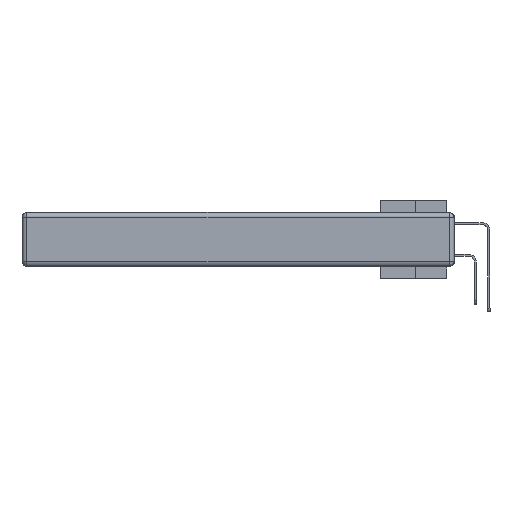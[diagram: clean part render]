
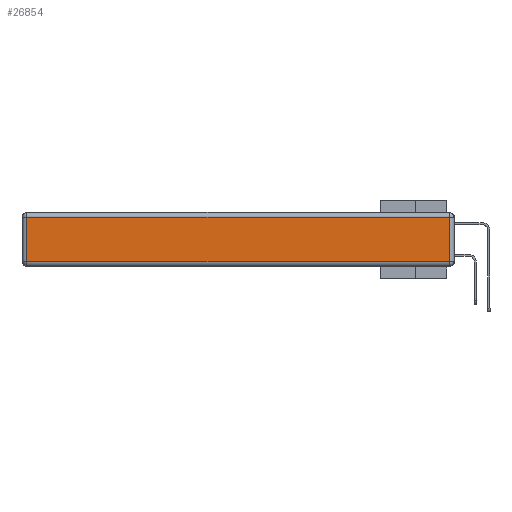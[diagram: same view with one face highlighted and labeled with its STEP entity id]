
A CAD part, left-side view. The second image highlights one B-rep face of the part: STEP entity #26854.
In plain terms, the highlighted planar face has unit normal (-1, 0, 0).
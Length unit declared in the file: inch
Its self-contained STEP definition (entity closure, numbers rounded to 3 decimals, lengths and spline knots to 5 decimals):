
#934 = VECTOR ( 'NONE', #37594, 39.37008 ) ;
#1810 = ORIENTED_EDGE ( 'NONE', *, *, #22919, .T. ) ;
#3829 = CARTESIAN_POINT ( 'NONE',  ( 0., 0.03, -0.03 ) ) ;
#5881 = FACE_OUTER_BOUND ( 'NONE', #35459, .T. ) ;
#6010 = CARTESIAN_POINT ( 'NONE',  ( 0., 2.72, -0.343 ) ) ;
#8460 = CARTESIAN_POINT ( 'NONE',  ( 0., 2.72, -0.03 ) ) ;
#8880 = CARTESIAN_POINT ( 'NONE',  ( 0., 0.03, -0.313 ) ) ;
#9746 = EDGE_CURVE ( 'NONE', #11923, #16937, #11888, .T. ) ;
#10973 = LINE ( 'NONE', #36894, #29405 ) ;
#11493 = DIRECTION ( 'NONE',  ( 0., -1., 0. ) ) ;
#11888 = LINE ( 'NONE', #37583, #28739 ) ;
#11923 = VERTEX_POINT ( 'NONE', #3829 ) ;
#13041 = PLANE ( 'NONE',  #17216 ) ;
#14494 = VECTOR ( 'NONE', #11493, 39.37008 ) ;
#15268 = DIRECTION ( 'NONE',  ( 0., 1., 0. ) ) ;
#16937 = VERTEX_POINT ( 'NONE', #8460 ) ;
#17216 = AXIS2_PLACEMENT_3D ( 'NONE', #31543, #19126, #37862 ) ;
#19126 = DIRECTION ( 'NONE',  ( -1., 0., 0. ) ) ;
#22044 = ORIENTED_EDGE ( 'NONE', *, *, #9746, .T. ) ;
#22919 = EDGE_CURVE ( 'NONE', #16937, #31050, #37797, .T. ) ;
#23920 = LINE ( 'NONE', #30861, #14494 ) ;
#24719 = CARTESIAN_POINT ( 'NONE',  ( 0., 2.72, -0.313 ) ) ;
#25894 = ORIENTED_EDGE ( 'NONE', *, *, #26064, .T. ) ;
#26064 = EDGE_CURVE ( 'NONE', #31050, #36430, #23920, .T. ) ;
#26854 = ADVANCED_FACE ( 'NONE', ( #5881 ), #13041, .T. ) ;
#28739 = VECTOR ( 'NONE', #15268, 39.37008 ) ;
#29405 = VECTOR ( 'NONE', #30779, 39.37008 ) ;
#29434 = EDGE_CURVE ( 'NONE', #36430, #11923, #10973, .T. ) ;
#30779 = DIRECTION ( 'NONE',  ( 0., 0., 1. ) ) ;
#30861 = CARTESIAN_POINT ( 'NONE',  ( 0., 0., -0.313 ) ) ;
#31050 = VERTEX_POINT ( 'NONE', #24719 ) ;
#31057 = ORIENTED_EDGE ( 'NONE', *, *, #29434, .T. ) ;
#31543 = CARTESIAN_POINT ( 'NONE',  ( 0., 0., -0.343 ) ) ;
#35459 = EDGE_LOOP ( 'NONE', ( #25894, #31057, #22044, #1810 ) ) ;
#36430 = VERTEX_POINT ( 'NONE', #8880 ) ;
#36894 = CARTESIAN_POINT ( 'NONE',  ( 0., 0.03, -0.343 ) ) ;
#37583 = CARTESIAN_POINT ( 'NONE',  ( 0., 2.75, -0.03 ) ) ;
#37594 = DIRECTION ( 'NONE',  ( 0., 0., -1. ) ) ;
#37797 = LINE ( 'NONE', #6010, #934 ) ;
#37862 = DIRECTION ( 'NONE',  ( 0., 0., 1. ) ) ;
